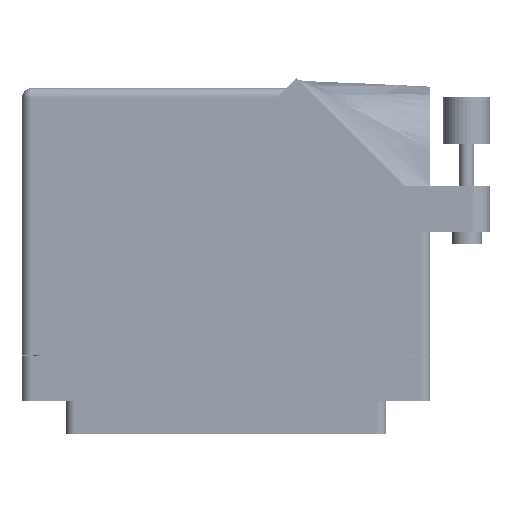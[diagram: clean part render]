
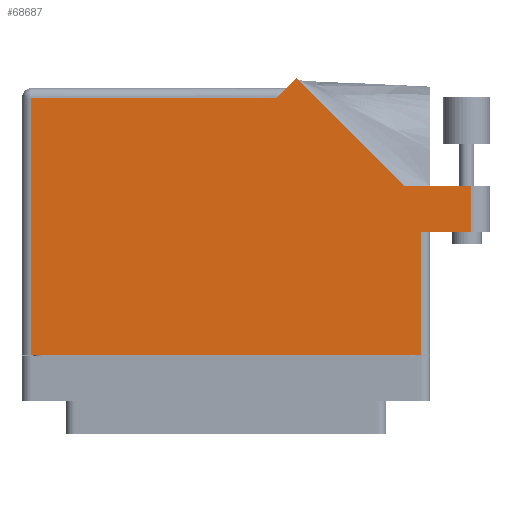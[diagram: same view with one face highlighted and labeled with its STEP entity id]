
A CAD part, front view. The second image highlights one B-rep face of the part: STEP entity #68687.
In plain terms, the highlighted face is planar.
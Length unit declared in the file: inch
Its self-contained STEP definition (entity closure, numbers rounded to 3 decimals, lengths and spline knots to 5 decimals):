
#540 = CARTESIAN_POINT ( 'NONE',  ( 1.634, 1.022, 0.617 ) ) ;
#2222 = LINE ( 'NONE', #13501, #48015 ) ;
#3144 = VERTEX_POINT ( 'NONE', #11254 ) ;
#4350 = VECTOR ( 'NONE', #22045, 39.37008 ) ;
#5235 = CARTESIAN_POINT ( 'NONE',  ( -1.297, -0.1, 0.617 ) ) ;
#6528 = CARTESIAN_POINT ( 'NONE',  ( -1.359, -0.1, 0.617 ) ) ;
#8614 = ORIENTED_EDGE ( 'NONE', *, *, #49717, .T. ) ;
#8624 = LINE ( 'NONE', #6528, #4350 ) ;
#10032 = CARTESIAN_POINT ( 'NONE',  ( 1.359, 0.715, 0.617 ) ) ;
#11254 = CARTESIAN_POINT ( 'NONE',  ( 1.19342, 1.022, 0.617 ) ) ;
#12398 = ORIENTED_EDGE ( 'NONE', *, *, #42091, .T. ) ;
#13501 = CARTESIAN_POINT ( 'NONE',  ( 1.19342, 1.022, 0.617 ) ) ;
#13567 = LINE ( 'NONE', #55413, #69614 ) ;
#16034 = EDGE_CURVE ( 'NONE', #59652, #58058, #8624, .T. ) ;
#17150 = VECTOR ( 'NONE', #44426, 39.37008 ) ;
#19043 = VECTOR ( 'NONE', #32576, 39.37008 ) ;
#21464 = VECTOR ( 'NONE', #68959, 39.37008 ) ;
#22045 = DIRECTION ( 'NONE',  ( 1., 0., 0. ) ) ;
#23252 = DIRECTION ( 'NONE',  ( -1., 0., 0. ) ) ;
#25029 = LINE ( 'NONE', #540, #19043 ) ;
#25718 = CARTESIAN_POINT ( 'NONE',  ( -1.297, -0.1, 0.617 ) ) ;
#26301 = CARTESIAN_POINT ( 'NONE',  ( 1.297, 0.715, 0.617 ) ) ;
#26716 = VECTOR ( 'NONE', #43210, 39.37008 ) ;
#27365 = EDGE_CURVE ( 'NONE', #63249, #59652, #65781, .T. ) ;
#28398 = CARTESIAN_POINT ( 'NONE',  ( 0.399, 1.675, 0.617 ) ) ;
#31632 = LINE ( 'NONE', #38996, #17150 ) ;
#32306 = DIRECTION ( 'NONE',  ( -1., 0., 0. ) ) ;
#32576 = DIRECTION ( 'NONE',  ( 0., 1., 0. ) ) ;
#34354 = EDGE_CURVE ( 'NONE', #58058, #39440, #13567, .T. ) ;
#34399 = FACE_OUTER_BOUND ( 'NONE', #55530, .T. ) ;
#35589 = DIRECTION ( 'NONE',  ( -0.707, 0.707, 0. ) ) ;
#36249 = VERTEX_POINT ( 'NONE', #44812 ) ;
#38996 = CARTESIAN_POINT ( 'NONE',  ( -1.359, 1.613, 0.617 ) ) ;
#39440 = VERTEX_POINT ( 'NONE', #26301 ) ;
#42091 = EDGE_CURVE ( 'NONE', #65245, #43132, #63569, .T. ) ;
#43132 = VERTEX_POINT ( 'NONE', #65358 ) ;
#43210 = DIRECTION ( 'NONE',  ( 0., -1., 0. ) ) ;
#43516 = ORIENTED_EDGE ( 'NONE', *, *, #27365, .T. ) ;
#44426 = DIRECTION ( 'NONE',  ( -1., 0., 0. ) ) ;
#44812 = CARTESIAN_POINT ( 'NONE',  ( 1.634, 1.022, 0.617 ) ) ;
#46083 = VECTOR ( 'NONE', #23252, 39.37008 ) ;
#47971 = DIRECTION ( 'NONE',  ( 0., 0., -1. ) ) ;
#48015 = VECTOR ( 'NONE', #35589, 39.37008 ) ;
#48137 = ORIENTED_EDGE ( 'NONE', *, *, #60295, .T. ) ;
#49717 = EDGE_CURVE ( 'NONE', #3144, #65245, #2222, .T. ) ;
#50197 = CARTESIAN_POINT ( 'NONE',  ( -1.297, 1.613, 0.617 ) ) ;
#50231 = LINE ( 'NONE', #10032, #21464 ) ;
#50781 = ORIENTED_EDGE ( 'NONE', *, *, #54637, .T. ) ;
#51630 = AXIS2_PLACEMENT_3D ( 'NONE', #59378, #47971, #32306 ) ;
#54488 = ORIENTED_EDGE ( 'NONE', *, *, #70320, .T. ) ;
#54535 = VERTEX_POINT ( 'NONE', #69340 ) ;
#54552 = LINE ( 'NONE', #67157, #46083 ) ;
#54637 = EDGE_CURVE ( 'NONE', #36249, #3144, #54552, .T. ) ;
#54682 = CARTESIAN_POINT ( 'NONE',  ( 0.46971, 1.74571, 0.617 ) ) ;
#55413 = CARTESIAN_POINT ( 'NONE',  ( 1.297, 0.715, 0.617 ) ) ;
#55530 = EDGE_LOOP ( 'NONE', ( #54488, #48137, #50781, #8614, #12398, #65213, #43516, #67873, #64559 ) ) ;
#58058 = VERTEX_POINT ( 'NONE', #62556 ) ;
#59378 = CARTESIAN_POINT ( 'NONE',  ( -1.359, 1.675, 0.617 ) ) ;
#59652 = VERTEX_POINT ( 'NONE', #5235 ) ;
#60295 = EDGE_CURVE ( 'NONE', #54535, #36249, #25029, .T. ) ;
#61872 = VECTOR ( 'NONE', #66118, 39.37008 ) ;
#62556 = CARTESIAN_POINT ( 'NONE',  ( 1.297, -0.1, 0.617 ) ) ;
#63249 = VERTEX_POINT ( 'NONE', #50197 ) ;
#63569 = LINE ( 'NONE', #28398, #61872 ) ;
#64559 = ORIENTED_EDGE ( 'NONE', *, *, #34354, .T. ) ;
#65213 = ORIENTED_EDGE ( 'NONE', *, *, #68484, .T. ) ;
#65245 = VERTEX_POINT ( 'NONE', #54682 ) ;
#65358 = CARTESIAN_POINT ( 'NONE',  ( 0.337, 1.613, 0.617 ) ) ;
#65433 = DIRECTION ( 'NONE',  ( 0., 1., 0. ) ) ;
#65781 = LINE ( 'NONE', #25718, #26716 ) ;
#66118 = DIRECTION ( 'NONE',  ( -0.707, -0.707, 0. ) ) ;
#67157 = CARTESIAN_POINT ( 'NONE',  ( 1.759, 1.022, 0.617 ) ) ;
#67873 = ORIENTED_EDGE ( 'NONE', *, *, #16034, .T. ) ;
#68484 = EDGE_CURVE ( 'NONE', #43132, #63249, #31632, .T. ) ;
#68687 = ADVANCED_FACE ( 'NONE', ( #34399 ), #70318, .F. ) ;
#68959 = DIRECTION ( 'NONE',  ( 1., 0., 0. ) ) ;
#69340 = CARTESIAN_POINT ( 'NONE',  ( 1.634, 0.715, 0.617 ) ) ;
#69614 = VECTOR ( 'NONE', #65433, 39.37008 ) ;
#70318 = PLANE ( 'NONE',  #51630 ) ;
#70320 = EDGE_CURVE ( 'NONE', #39440, #54535, #50231, .T. ) ;
